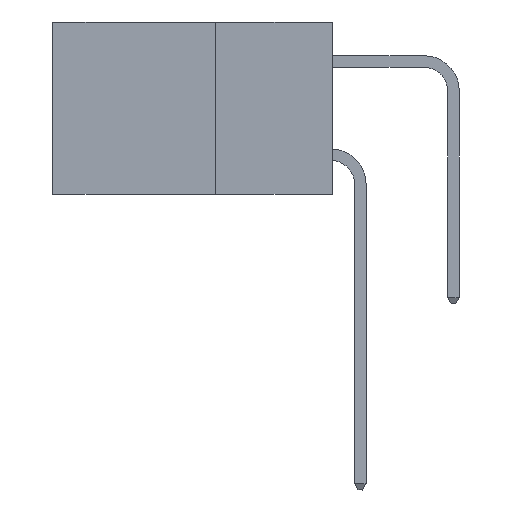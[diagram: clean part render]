
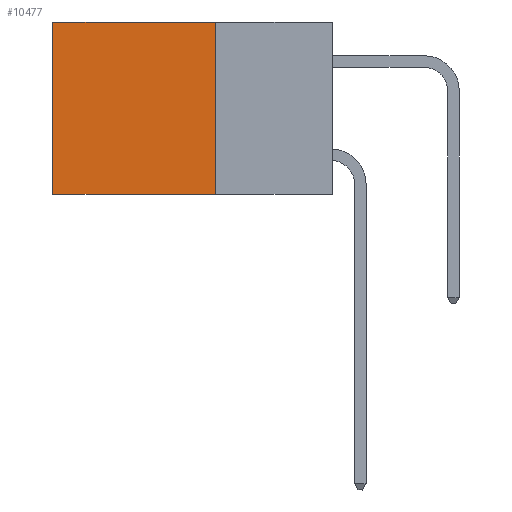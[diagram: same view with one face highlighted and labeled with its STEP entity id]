
A CAD part, left-side view. The second image highlights one B-rep face of the part: STEP entity #10477.
In plain terms, the highlighted planar face has unit normal (-1, 0, 0).
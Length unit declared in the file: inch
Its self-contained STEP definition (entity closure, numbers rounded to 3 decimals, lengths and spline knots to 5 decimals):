
#929 = LINE ( 'NONE', #5456, #19338 ) ;
#2345 = LINE ( 'NONE', #4328, #12368 ) ;
#3017 = VERTEX_POINT ( 'NONE', #23103 ) ;
#4328 = CARTESIAN_POINT ( 'NONE',  ( 0.2615, 0.25, -0.37 ) ) ;
#5118 = EDGE_CURVE ( 'NONE', #19442, #3017, #929, .T. ) ;
#5456 = CARTESIAN_POINT ( 'NONE',  ( 0.2615, 0.25, -0.37 ) ) ;
#6639 = DIRECTION ( 'NONE',  ( 0., 0., -1. ) ) ;
#7790 = CARTESIAN_POINT ( 'NONE',  ( 0.2615, 0.25, 0. ) ) ;
#8742 = CARTESIAN_POINT ( 'NONE',  ( 0.2615, 0.25, 0. ) ) ;
#9467 = AXIS2_PLACEMENT_3D ( 'NONE', #15519, #21585, #6639 ) ;
#10477 = ADVANCED_FACE ( 'NONE', ( #17344 ), #13263, .F. ) ;
#11203 = LINE ( 'NONE', #20574, #21043 ) ;
#12264 = VERTEX_POINT ( 'NONE', #27503 ) ;
#12368 = VECTOR ( 'NONE', #15320, 39.37008 ) ;
#12872 = EDGE_CURVE ( 'NONE', #20739, #19442, #2345, .T. ) ;
#12940 = EDGE_LOOP ( 'NONE', ( #25527, #27747, #23513, #16814 ) ) ;
#13263 = PLANE ( 'NONE',  #9467 ) ;
#13988 = DIRECTION ( 'NONE',  ( 0., 1., 0. ) ) ;
#14112 = DIRECTION ( 'NONE',  ( 0., 0., -1. ) ) ;
#15057 = CARTESIAN_POINT ( 'NONE',  ( 0.2615, 0.25, -0.37 ) ) ;
#15320 = DIRECTION ( 'NONE',  ( 0., 0., -1. ) ) ;
#15519 = CARTESIAN_POINT ( 'NONE',  ( 0.2615, 0.25, -0.37 ) ) ;
#16814 = ORIENTED_EDGE ( 'NONE', *, *, #18771, .T. ) ;
#17344 = FACE_OUTER_BOUND ( 'NONE', #12940, .T. ) ;
#18487 = VECTOR ( 'NONE', #13988, 39.37008 ) ;
#18615 = LINE ( 'NONE', #7790, #18487 ) ;
#18771 = EDGE_CURVE ( 'NONE', #20739, #12264, #18615, .T. ) ;
#19338 = VECTOR ( 'NONE', #26583, 39.37008 ) ;
#19442 = VERTEX_POINT ( 'NONE', #15057 ) ;
#20574 = CARTESIAN_POINT ( 'NONE',  ( 0.2615, 0.6, -0.37 ) ) ;
#20739 = VERTEX_POINT ( 'NONE', #8742 ) ;
#21043 = VECTOR ( 'NONE', #14112, 39.37008 ) ;
#21585 = DIRECTION ( 'NONE',  ( 1., 0., 0. ) ) ;
#23103 = CARTESIAN_POINT ( 'NONE',  ( 0.2615, 0.6, -0.37 ) ) ;
#23513 = ORIENTED_EDGE ( 'NONE', *, *, #12872, .F. ) ;
#25527 = ORIENTED_EDGE ( 'NONE', *, *, #27498, .T. ) ;
#26583 = DIRECTION ( 'NONE',  ( 0., 1., 0. ) ) ;
#27498 = EDGE_CURVE ( 'NONE', #12264, #3017, #11203, .T. ) ;
#27503 = CARTESIAN_POINT ( 'NONE',  ( 0.2615, 0.6, 0. ) ) ;
#27747 = ORIENTED_EDGE ( 'NONE', *, *, #5118, .F. ) ;
